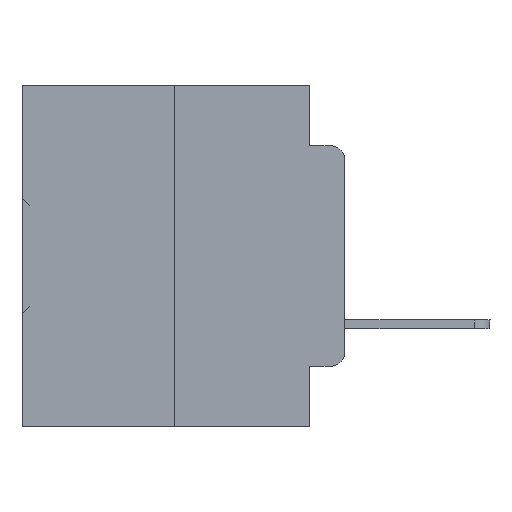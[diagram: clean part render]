
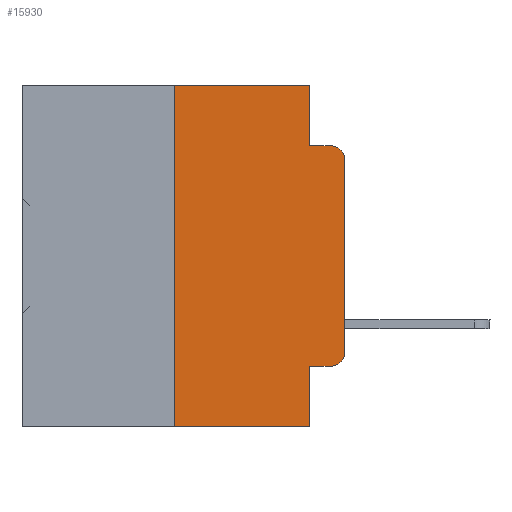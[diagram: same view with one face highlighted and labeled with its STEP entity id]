
A CAD part, left-side view. The second image highlights one B-rep face of the part: STEP entity #15930.
In plain terms, the highlighted planar face has unit normal (-1, 0, 0).
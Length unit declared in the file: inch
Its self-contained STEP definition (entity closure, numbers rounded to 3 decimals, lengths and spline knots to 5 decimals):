
#217 = LINE ( 'NONE', #14826, #26017 ) ;
#413 = DIRECTION ( 'NONE',  ( -1., 0., 0. ) ) ;
#841 = AXIS2_PLACEMENT_3D ( 'NONE', #22264, #11248, #25645 ) ;
#1389 = EDGE_LOOP ( 'NONE', ( #7248, #33813, #13754, #6750, #17800, #2995, #31678, #25662, #5247, #35542 ) ) ;
#1633 = EDGE_CURVE ( 'NONE', #18616, #15751, #20114, .T. ) ;
#1988 = VECTOR ( 'NONE', #16129, 39.37008 ) ;
#2356 = CARTESIAN_POINT ( 'NONE',  ( 0., 0.051, 0. ) ) ;
#2828 = DIRECTION ( 'NONE',  ( 0., 0., -1. ) ) ;
#2881 = VERTEX_POINT ( 'NONE', #15578 ) ;
#2995 = ORIENTED_EDGE ( 'NONE', *, *, #10766, .F. ) ;
#3006 = LINE ( 'NONE', #8899, #33437 ) ;
#3334 = CARTESIAN_POINT ( 'NONE',  ( 0., 0.02, -0.3915 ) ) ;
#4332 = EDGE_CURVE ( 'NONE', #22327, #17937, #27344, .T. ) ;
#4647 = CARTESIAN_POINT ( 'NONE',  ( 0., 0.051, -0.0885 ) ) ;
#4958 = DIRECTION ( 'NONE',  ( 0., 0., -1. ) ) ;
#5172 = VECTOR ( 'NONE', #31615, 39.37008 ) ;
#5247 = ORIENTED_EDGE ( 'NONE', *, *, #15650, .T. ) ;
#5877 = VERTEX_POINT ( 'NONE', #2356 ) ;
#5950 = VERTEX_POINT ( 'NONE', #10423 ) ;
#6165 = EDGE_CURVE ( 'NONE', #9494, #17937, #3006, .T. ) ;
#6750 = ORIENTED_EDGE ( 'NONE', *, *, #30023, .F. ) ;
#7248 = ORIENTED_EDGE ( 'NONE', *, *, #36015, .T. ) ;
#7402 = CARTESIAN_POINT ( 'NONE',  ( 0., 0.051, -0.4115 ) ) ;
#8899 = CARTESIAN_POINT ( 'NONE',  ( 0., 0.051, 0. ) ) ;
#9494 = VERTEX_POINT ( 'NONE', #35003 ) ;
#9569 = DIRECTION ( 'NONE',  ( -1., 0., 0. ) ) ;
#10393 = CARTESIAN_POINT ( 'NONE',  ( 0., 0.25, -0.5 ) ) ;
#10423 = CARTESIAN_POINT ( 'NONE',  ( 0., 0.25, 0. ) ) ;
#10766 = EDGE_CURVE ( 'NONE', #22327, #5950, #217, .T. ) ;
#10866 = FACE_OUTER_BOUND ( 'NONE', #1389, .T. ) ;
#11248 = DIRECTION ( 'NONE',  ( 1., 0., 0. ) ) ;
#11291 = AXIS2_PLACEMENT_3D ( 'NONE', #3334, #9569, #32135 ) ;
#12773 = VERTEX_POINT ( 'NONE', #26495 ) ;
#13702 = CIRCLE ( 'NONE', #11291, 0.02 ) ;
#13754 = ORIENTED_EDGE ( 'NONE', *, *, #26482, .F. ) ;
#14732 = VECTOR ( 'NONE', #30150, 39.37008 ) ;
#14826 = CARTESIAN_POINT ( 'NONE',  ( 0., 0.25, 0. ) ) ;
#15578 = CARTESIAN_POINT ( 'NONE',  ( 0., 0.02, -0.4115 ) ) ;
#15650 = EDGE_CURVE ( 'NONE', #9494, #2881, #19852, .T. ) ;
#15751 = VERTEX_POINT ( 'NONE', #28931 ) ;
#15930 = ADVANCED_FACE ( 'NONE', ( #10866 ), #33962, .F. ) ;
#16129 = DIRECTION ( 'NONE',  ( 0., 0., 1. ) ) ;
#17755 = CARTESIAN_POINT ( 'NONE',  ( 0., 0.051, -0.5 ) ) ;
#17800 = ORIENTED_EDGE ( 'NONE', *, *, #26300, .F. ) ;
#17937 = VERTEX_POINT ( 'NONE', #17755 ) ;
#18363 = CARTESIAN_POINT ( 'NONE',  ( 0., 0.051, -0.0885 ) ) ;
#18616 = VERTEX_POINT ( 'NONE', #36771 ) ;
#19852 = LINE ( 'NONE', #7402, #14732 ) ;
#20114 = CIRCLE ( 'NONE', #29787, 0.02 ) ;
#21595 = VERTEX_POINT ( 'NONE', #4647 ) ;
#22264 = CARTESIAN_POINT ( 'NONE',  ( 0., 0.473, 0. ) ) ;
#22327 = VERTEX_POINT ( 'NONE', #10393 ) ;
#22797 = CARTESIAN_POINT ( 'NONE',  ( 0., 0.051, 0. ) ) ;
#25645 = DIRECTION ( 'NONE',  ( 0., 0., -1. ) ) ;
#25662 = ORIENTED_EDGE ( 'NONE', *, *, #6165, .F. ) ;
#26017 = VECTOR ( 'NONE', #34296, 39.37008 ) ;
#26300 = EDGE_CURVE ( 'NONE', #5950, #5877, #31989, .T. ) ;
#26482 = EDGE_CURVE ( 'NONE', #21595, #15751, #29712, .T. ) ;
#26495 = CARTESIAN_POINT ( 'NONE',  ( 0., 0., -0.3915 ) ) ;
#26590 = VECTOR ( 'NONE', #4958, 39.37008 ) ;
#26926 = EDGE_CURVE ( 'NONE', #2881, #12773, #13702, .T. ) ;
#27344 = LINE ( 'NONE', #36224, #32087 ) ;
#27714 = DIRECTION ( 'NONE',  ( 0., -1., 0. ) ) ;
#28931 = CARTESIAN_POINT ( 'NONE',  ( 0., 0.02, -0.0885 ) ) ;
#29202 = CARTESIAN_POINT ( 'NONE',  ( 0., 0.02, -0.1085 ) ) ;
#29712 = LINE ( 'NONE', #18363, #30017 ) ;
#29787 = AXIS2_PLACEMENT_3D ( 'NONE', #29202, #413, #35246 ) ;
#30017 = VECTOR ( 'NONE', #35947, 39.37008 ) ;
#30023 = EDGE_CURVE ( 'NONE', #5877, #21595, #30928, .T. ) ;
#30150 = DIRECTION ( 'NONE',  ( 0., -1., 0. ) ) ;
#30928 = LINE ( 'NONE', #22797, #26590 ) ;
#31615 = DIRECTION ( 'NONE',  ( 0., -1., 0. ) ) ;
#31678 = ORIENTED_EDGE ( 'NONE', *, *, #4332, .T. ) ;
#31989 = LINE ( 'NONE', #34437, #5172 ) ;
#32087 = VECTOR ( 'NONE', #27714, 39.37008 ) ;
#32135 = DIRECTION ( 'NONE',  ( 0., 0., -1. ) ) ;
#33152 = LINE ( 'NONE', #35995, #1988 ) ;
#33437 = VECTOR ( 'NONE', #2828, 39.37008 ) ;
#33813 = ORIENTED_EDGE ( 'NONE', *, *, #1633, .T. ) ;
#33962 = PLANE ( 'NONE',  #841 ) ;
#34296 = DIRECTION ( 'NONE',  ( 0., 0., 1. ) ) ;
#34437 = CARTESIAN_POINT ( 'NONE',  ( 0., 0.473, 0. ) ) ;
#35003 = CARTESIAN_POINT ( 'NONE',  ( 0., 0.051, -0.4115 ) ) ;
#35246 = DIRECTION ( 'NONE',  ( 0., 0., -1. ) ) ;
#35542 = ORIENTED_EDGE ( 'NONE', *, *, #26926, .T. ) ;
#35947 = DIRECTION ( 'NONE',  ( 0., -1., 0. ) ) ;
#35995 = CARTESIAN_POINT ( 'NONE',  ( 0., 0., 0. ) ) ;
#36015 = EDGE_CURVE ( 'NONE', #12773, #18616, #33152, .T. ) ;
#36224 = CARTESIAN_POINT ( 'NONE',  ( 0., 0.473, -0.5 ) ) ;
#36771 = CARTESIAN_POINT ( 'NONE',  ( 0., 0., -0.1085 ) ) ;
